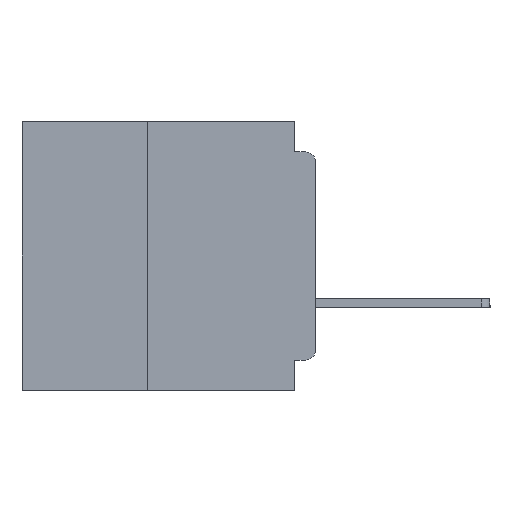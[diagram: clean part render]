
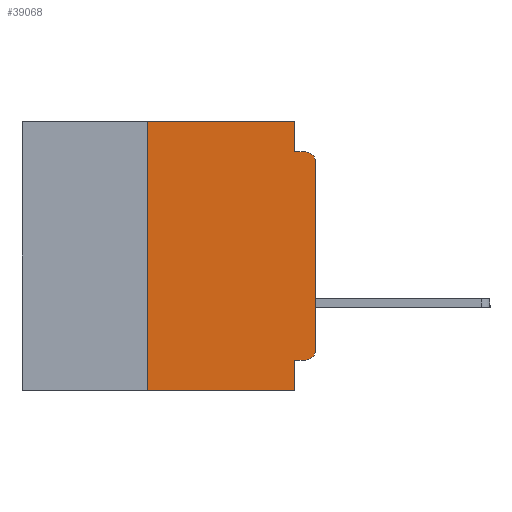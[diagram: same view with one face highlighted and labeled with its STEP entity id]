
A CAD part, left-side view. The second image highlights one B-rep face of the part: STEP entity #39068.
In plain terms, the highlighted planar face has unit normal (-1, 0, 0).
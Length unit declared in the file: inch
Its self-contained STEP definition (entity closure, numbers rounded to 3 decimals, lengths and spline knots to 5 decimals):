
#1265 = CARTESIAN_POINT ( 'NONE',  ( 0., 0.015, -0.06 ) ) ;
#1300 = ORIENTED_EDGE ( 'NONE', *, *, #26481, .F. ) ;
#1626 = LINE ( 'NONE', #30244, #10134 ) ;
#1795 = VECTOR ( 'NONE', #41317, 39.37008 ) ;
#1957 = DIRECTION ( 'NONE',  ( 0., -1., 0. ) ) ;
#2049 = VERTEX_POINT ( 'NONE', #18844 ) ;
#2388 = ORIENTED_EDGE ( 'NONE', *, *, #43609, .T. ) ;
#2842 = EDGE_CURVE ( 'NONE', #5614, #16361, #23185, .T. ) ;
#3578 = LINE ( 'NONE', #30626, #31041 ) ;
#3617 = ORIENTED_EDGE ( 'NONE', *, *, #2842, .F. ) ;
#4384 = EDGE_CURVE ( 'NONE', #26705, #9227, #25562, .T. ) ;
#4917 = DIRECTION ( 'NONE',  ( 0., 0., -1. ) ) ;
#5117 = DIRECTION ( 'NONE',  ( 0., -1., 0. ) ) ;
#5427 = FACE_OUTER_BOUND ( 'NONE', #40546, .T. ) ;
#5614 = VERTEX_POINT ( 'NONE', #39138 ) ;
#5684 = CARTESIAN_POINT ( 'NONE',  ( 0., 0., -0.045 ) ) ;
#5941 = CARTESIAN_POINT ( 'NONE',  ( 0., 0.437, 0. ) ) ;
#6252 = EDGE_CURVE ( 'NONE', #16361, #2049, #20871, .T. ) ;
#8016 = CARTESIAN_POINT ( 'NONE',  ( 0., 0.25, -0.4 ) ) ;
#9227 = VERTEX_POINT ( 'NONE', #40734 ) ;
#9610 = DIRECTION ( 'NONE',  ( 0., 0., -1. ) ) ;
#10134 = VECTOR ( 'NONE', #12481, 39.37008 ) ;
#11659 = DIRECTION ( 'NONE',  ( 0., 0., 1. ) ) ;
#12194 = CIRCLE ( 'NONE', #22791, 0.015 ) ;
#12481 = DIRECTION ( 'NONE',  ( 0., 0., 1. ) ) ;
#12598 = DIRECTION ( 'NONE',  ( 0., -1., 0. ) ) ;
#12654 = ORIENTED_EDGE ( 'NONE', *, *, #6252, .F. ) ;
#13671 = VECTOR ( 'NONE', #11659, 39.37008 ) ;
#14457 = VECTOR ( 'NONE', #32485, 39.37008 ) ;
#14648 = CARTESIAN_POINT ( 'NONE',  ( 0., 0., -0.34 ) ) ;
#15428 = AXIS2_PLACEMENT_3D ( 'NONE', #21024, #45962, #24630 ) ;
#15555 = LINE ( 'NONE', #42927, #14457 ) ;
#15867 = CARTESIAN_POINT ( 'NONE',  ( 0., 0.031, 0. ) ) ;
#16183 = CARTESIAN_POINT ( 'NONE',  ( 0., 0.031, -0.045 ) ) ;
#16361 = VERTEX_POINT ( 'NONE', #25538 ) ;
#17587 = EDGE_CURVE ( 'NONE', #31164, #9227, #12194, .T. ) ;
#18844 = CARTESIAN_POINT ( 'NONE',  ( 0., 0.031, -0.4 ) ) ;
#19882 = EDGE_CURVE ( 'NONE', #42948, #21310, #21451, .T. ) ;
#20871 = LINE ( 'NONE', #41715, #1795 ) ;
#21024 = CARTESIAN_POINT ( 'NONE',  ( 0., 0.015, -0.34 ) ) ;
#21310 = VERTEX_POINT ( 'NONE', #15867 ) ;
#21451 = LINE ( 'NONE', #30361, #29866 ) ;
#22066 = VECTOR ( 'NONE', #39821, 39.37008 ) ;
#22791 = AXIS2_PLACEMENT_3D ( 'NONE', #1265, #26376, #4917 ) ;
#22976 = VERTEX_POINT ( 'NONE', #14648 ) ;
#23185 = LINE ( 'NONE', #24550, #22066 ) ;
#24275 = ORIENTED_EDGE ( 'NONE', *, *, #45767, .F. ) ;
#24550 = CARTESIAN_POINT ( 'NONE',  ( 0., 0., -0.355 ) ) ;
#24630 = DIRECTION ( 'NONE',  ( 0., 0., -1. ) ) ;
#24751 = EDGE_CURVE ( 'NONE', #34059, #2049, #3578, .T. ) ;
#25538 = CARTESIAN_POINT ( 'NONE',  ( 0., 0.031, -0.355 ) ) ;
#25562 = LINE ( 'NONE', #5684, #35053 ) ;
#26106 = CARTESIAN_POINT ( 'NONE',  ( 0., 0.25, 0. ) ) ;
#26376 = DIRECTION ( 'NONE',  ( -1., 0., 0. ) ) ;
#26481 = EDGE_CURVE ( 'NONE', #34059, #42948, #32631, .T. ) ;
#26705 = VERTEX_POINT ( 'NONE', #16183 ) ;
#28196 = ORIENTED_EDGE ( 'NONE', *, *, #4384, .F. ) ;
#29866 = VECTOR ( 'NONE', #12598, 39.37008 ) ;
#30244 = CARTESIAN_POINT ( 'NONE',  ( 0., 0., 0. ) ) ;
#30361 = CARTESIAN_POINT ( 'NONE',  ( 0., 0.437, 0. ) ) ;
#30626 = CARTESIAN_POINT ( 'NONE',  ( 0., 0.437, -0.4 ) ) ;
#30965 = DIRECTION ( 'NONE',  ( 1., 0., 0. ) ) ;
#31041 = VECTOR ( 'NONE', #1957, 39.37008 ) ;
#31164 = VERTEX_POINT ( 'NONE', #46014 ) ;
#32485 = DIRECTION ( 'NONE',  ( 0., 0., -1. ) ) ;
#32631 = LINE ( 'NONE', #8016, #13671 ) ;
#33281 = ORIENTED_EDGE ( 'NONE', *, *, #24751, .T. ) ;
#33935 = EDGE_CURVE ( 'NONE', #5614, #22976, #43550, .T. ) ;
#34059 = VERTEX_POINT ( 'NONE', #43047 ) ;
#34916 = ORIENTED_EDGE ( 'NONE', *, *, #19882, .F. ) ;
#35053 = VECTOR ( 'NONE', #5117, 39.37008 ) ;
#35551 = ORIENTED_EDGE ( 'NONE', *, *, #33935, .T. ) ;
#39068 = ADVANCED_FACE ( 'NONE', ( #5427 ), #45133, .F. ) ;
#39138 = CARTESIAN_POINT ( 'NONE',  ( 0., 0.015, -0.355 ) ) ;
#39821 = DIRECTION ( 'NONE',  ( 0., 1., 0. ) ) ;
#40546 = EDGE_LOOP ( 'NONE', ( #2388, #46009, #28196, #24275, #34916, #1300, #33281, #12654, #3617, #35551 ) ) ;
#40734 = CARTESIAN_POINT ( 'NONE',  ( 0., 0.015, -0.045 ) ) ;
#40893 = AXIS2_PLACEMENT_3D ( 'NONE', #5941, #30965, #9610 ) ;
#41317 = DIRECTION ( 'NONE',  ( 0., 0., -1. ) ) ;
#41715 = CARTESIAN_POINT ( 'NONE',  ( 0., 0.031, -0.4 ) ) ;
#42927 = CARTESIAN_POINT ( 'NONE',  ( 0., 0.031, 0. ) ) ;
#42948 = VERTEX_POINT ( 'NONE', #26106 ) ;
#43047 = CARTESIAN_POINT ( 'NONE',  ( 0., 0.25, -0.4 ) ) ;
#43550 = CIRCLE ( 'NONE', #15428, 0.015 ) ;
#43609 = EDGE_CURVE ( 'NONE', #22976, #31164, #1626, .T. ) ;
#45133 = PLANE ( 'NONE',  #40893 ) ;
#45767 = EDGE_CURVE ( 'NONE', #21310, #26705, #15555, .T. ) ;
#45962 = DIRECTION ( 'NONE',  ( -1., 0., 0. ) ) ;
#46009 = ORIENTED_EDGE ( 'NONE', *, *, #17587, .T. ) ;
#46014 = CARTESIAN_POINT ( 'NONE',  ( 0., 0., -0.06 ) ) ;
